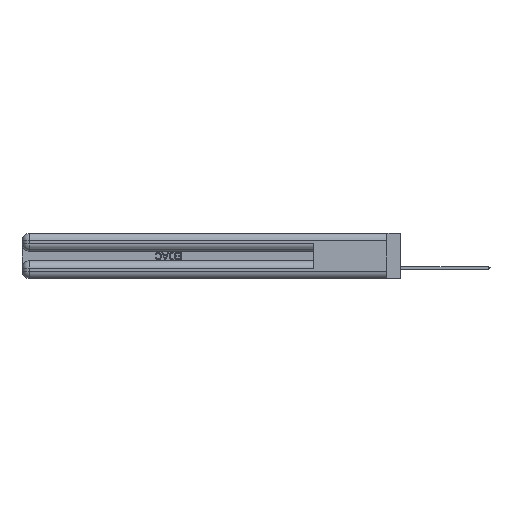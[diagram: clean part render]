
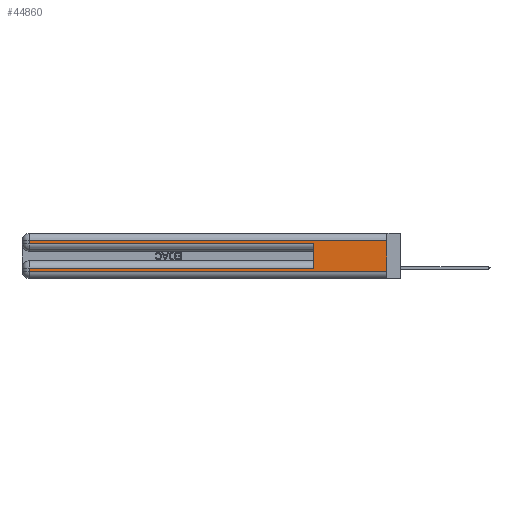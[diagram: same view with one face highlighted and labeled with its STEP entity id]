
A CAD part, left-side view. The second image highlights one B-rep face of the part: STEP entity #44860.
In plain terms, the highlighted planar face has unit normal (-1, 0, 0).
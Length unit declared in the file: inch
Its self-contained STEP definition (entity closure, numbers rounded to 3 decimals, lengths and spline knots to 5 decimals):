
#311 = VECTOR ( 'NONE', #29578, 39.37008 ) ;
#850 = EDGE_CURVE ( 'NONE', #38122, #11913, #1652, .T. ) ;
#1350 = CARTESIAN_POINT ( 'NONE',  ( 0., 0.6, 0.285 ) ) ;
#1425 = LINE ( 'NONE', #11224, #311 ) ;
#1652 = LINE ( 'NONE', #1924, #39327 ) ;
#1924 = CARTESIAN_POINT ( 'NONE',  ( 0., 0., 0.31 ) ) ;
#2945 = LINE ( 'NONE', #40742, #8626 ) ;
#3119 = ORIENTED_EDGE ( 'NONE', *, *, #9692, .T. ) ;
#4190 = VERTEX_POINT ( 'NONE', #46253 ) ;
#4248 = DIRECTION ( 'NONE',  ( 0., 0., -1. ) ) ;
#5160 = CARTESIAN_POINT ( 'NONE',  ( 0., 2.94, 0.37 ) ) ;
#6095 = LINE ( 'NONE', #46778, #36362 ) ;
#6728 = DIRECTION ( 'NONE',  ( 1., 0., 0. ) ) ;
#6963 = VERTEX_POINT ( 'NONE', #38708 ) ;
#7043 = DIRECTION ( 'NONE',  ( 0., 0., -1. ) ) ;
#7054 = EDGE_LOOP ( 'NONE', ( #30480, #43011, #7573, #26151, #24056, #3119, #26663, #15980 ) ) ;
#7573 = ORIENTED_EDGE ( 'NONE', *, *, #40512, .T. ) ;
#7820 = EDGE_CURVE ( 'NONE', #36024, #14139, #1425, .T. ) ;
#8626 = VECTOR ( 'NONE', #4248, 39.37008 ) ;
#8819 = DIRECTION ( 'NONE',  ( 0., 0., -1. ) ) ;
#9692 = EDGE_CURVE ( 'NONE', #6963, #11991, #24616, .T. ) ;
#10093 = VECTOR ( 'NONE', #8819, 39.37008 ) ;
#11052 = EDGE_CURVE ( 'NONE', #4190, #43348, #35410, .T. ) ;
#11224 = CARTESIAN_POINT ( 'NONE',  ( 0., 0., 0.285 ) ) ;
#11913 = VERTEX_POINT ( 'NONE', #33548 ) ;
#11991 = VERTEX_POINT ( 'NONE', #35840 ) ;
#13666 = CARTESIAN_POINT ( 'NONE',  ( 0., 0., 0.06 ) ) ;
#13903 = EDGE_CURVE ( 'NONE', #6963, #14139, #25452, .T. ) ;
#14139 = VERTEX_POINT ( 'NONE', #1350 ) ;
#15534 = CARTESIAN_POINT ( 'NONE',  ( 0., 2.94, 0.285 ) ) ;
#15980 = ORIENTED_EDGE ( 'NONE', *, *, #11052, .T. ) ;
#16051 = DIRECTION ( 'NONE',  ( 0., 1., 0. ) ) ;
#17430 = CARTESIAN_POINT ( 'NONE',  ( 0., 0., 0.37 ) ) ;
#21797 = DIRECTION ( 'NONE',  ( 0., 0., -1. ) ) ;
#21975 = CARTESIAN_POINT ( 'NONE',  ( 0., 0.6, 0.145 ) ) ;
#22615 = VECTOR ( 'NONE', #36486, 39.37008 ) ;
#24056 = ORIENTED_EDGE ( 'NONE', *, *, #13903, .F. ) ;
#24450 = CARTESIAN_POINT ( 'NONE',  ( 0., 0., 0.06 ) ) ;
#24616 = LINE ( 'NONE', #30706, #41783 ) ;
#25452 = LINE ( 'NONE', #21975, #22615 ) ;
#26151 = ORIENTED_EDGE ( 'NONE', *, *, #7820, .T. ) ;
#26663 = ORIENTED_EDGE ( 'NONE', *, *, #35016, .T. ) ;
#28579 = PLANE ( 'NONE',  #43139 ) ;
#29578 = DIRECTION ( 'NONE',  ( 0., -1., 0. ) ) ;
#30480 = ORIENTED_EDGE ( 'NONE', *, *, #37060, .F. ) ;
#30706 = CARTESIAN_POINT ( 'NONE',  ( 0., 0., 0.085 ) ) ;
#33548 = CARTESIAN_POINT ( 'NONE',  ( 0., 2.94, 0.31 ) ) ;
#35016 = EDGE_CURVE ( 'NONE', #11991, #4190, #46592, .T. ) ;
#35048 = FACE_OUTER_BOUND ( 'NONE', #7054, .T. ) ;
#35410 = LINE ( 'NONE', #13666, #43936 ) ;
#35840 = CARTESIAN_POINT ( 'NONE',  ( 0., 2.94, 0.085 ) ) ;
#36024 = VERTEX_POINT ( 'NONE', #15534 ) ;
#36362 = VECTOR ( 'NONE', #21797, 39.37008 ) ;
#36486 = DIRECTION ( 'NONE',  ( 0., 0., 1. ) ) ;
#37060 = EDGE_CURVE ( 'NONE', #38122, #43348, #6095, .T. ) ;
#38122 = VERTEX_POINT ( 'NONE', #41934 ) ;
#38708 = CARTESIAN_POINT ( 'NONE',  ( 0., 0.6, 0.085 ) ) ;
#38759 = DIRECTION ( 'NONE',  ( 0., 1., 0. ) ) ;
#39164 = DIRECTION ( 'NONE',  ( 0., -1., 0. ) ) ;
#39327 = VECTOR ( 'NONE', #38759, 39.37008 ) ;
#40512 = EDGE_CURVE ( 'NONE', #11913, #36024, #2945, .T. ) ;
#40742 = CARTESIAN_POINT ( 'NONE',  ( 0., 2.94, 0.37 ) ) ;
#41783 = VECTOR ( 'NONE', #16051, 39.37008 ) ;
#41934 = CARTESIAN_POINT ( 'NONE',  ( 0., 0., 0.31 ) ) ;
#43011 = ORIENTED_EDGE ( 'NONE', *, *, #850, .T. ) ;
#43139 = AXIS2_PLACEMENT_3D ( 'NONE', #17430, #6728, #7043 ) ;
#43348 = VERTEX_POINT ( 'NONE', #24450 ) ;
#43936 = VECTOR ( 'NONE', #39164, 39.37008 ) ;
#44860 = ADVANCED_FACE ( 'NONE', ( #35048 ), #28579, .F. ) ;
#46253 = CARTESIAN_POINT ( 'NONE',  ( 0., 2.94, 0.06 ) ) ;
#46592 = LINE ( 'NONE', #5160, #10093 ) ;
#46778 = CARTESIAN_POINT ( 'NONE',  ( 0., 0., 0.37 ) ) ;
